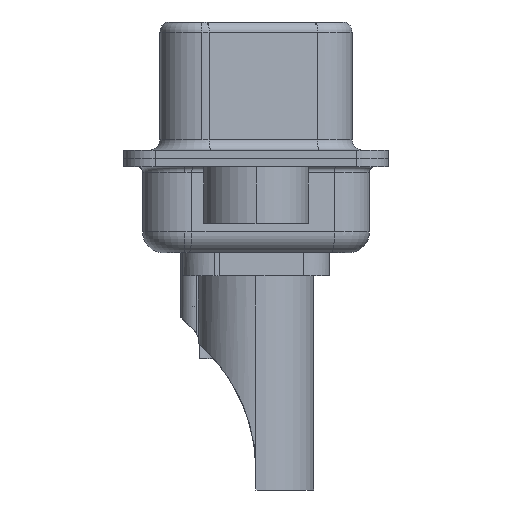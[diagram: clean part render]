
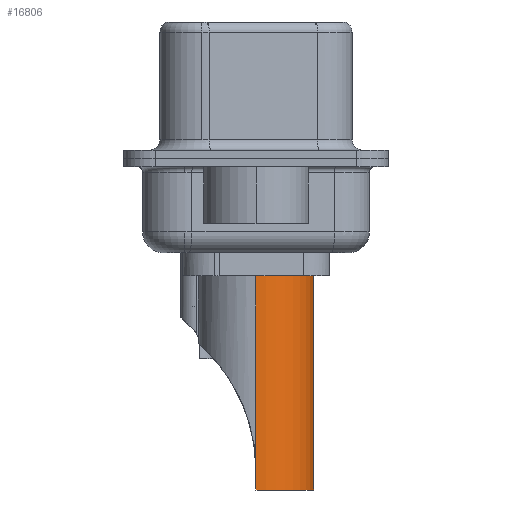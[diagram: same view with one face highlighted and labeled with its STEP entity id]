
A CAD part, left-side view. The second image highlights one B-rep face of the part: STEP entity #16806.
In plain terms, the highlighted cylindrical face has radius 2.75 mm (diameter 5.5 mm), a partial arc.
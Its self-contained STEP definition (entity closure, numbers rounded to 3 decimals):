
#46 = CARTESIAN_POINT ( 'NONE',  ( -2.75, 0., -8.7 ) ) ;
#313 = DIRECTION ( 'NONE',  ( 1., 0., 0. ) ) ;
#551 = VECTOR ( 'NONE', #22074, 1000. ) ;
#623 = VERTEX_POINT ( 'NONE', #10747 ) ;
#1064 = VERTEX_POINT ( 'NONE', #5358 ) ;
#1461 = EDGE_CURVE ( 'NONE', #8605, #7674, #19574, .T. ) ;
#1521 = VECTOR ( 'NONE', #18967, 1000. ) ;
#2049 = EDGE_CURVE ( 'NONE', #623, #7674, #20118, .T. ) ;
#2072 = DIRECTION ( 'NONE',  ( 0., 0., 1. ) ) ;
#3609 = CYLINDRICAL_SURFACE ( 'NONE', #22274, 2.75 ) ;
#4713 = ORIENTED_EDGE ( 'NONE', *, *, #18797, .T. ) ;
#4918 = LINE ( 'NONE', #21689, #9690 ) ;
#4948 = DIRECTION ( 'NONE',  ( 0., 0., 1. ) ) ;
#5270 = LINE ( 'NONE', #18436, #551 ) ;
#5358 = CARTESIAN_POINT ( 'NONE',  ( -2.75, 0., -7.764 ) ) ;
#5475 = DIRECTION ( 'NONE',  ( 0., 0., -1. ) ) ;
#7674 = VERTEX_POINT ( 'NONE', #19712 ) ;
#7892 = EDGE_CURVE ( 'NONE', #623, #22206, #5270, .T. ) ;
#8605 = VERTEX_POINT ( 'NONE', #18843 ) ;
#8950 = FACE_OUTER_BOUND ( 'NONE', #19114, .T. ) ;
#9690 = VECTOR ( 'NONE', #5475, 1000. ) ;
#9710 = ORIENTED_EDGE ( 'NONE', *, *, #7892, .F. ) ;
#9811 = CARTESIAN_POINT ( 'NONE',  ( -2.75, 0., 4.234 ) ) ;
#9864 = DIRECTION ( 'NONE',  ( 0., 0., 1. ) ) ;
#9958 = ORIENTED_EDGE ( 'NONE', *, *, #2049, .T. ) ;
#10747 = CARTESIAN_POINT ( 'NONE',  ( 2.75, 0., -7.764 ) ) ;
#11402 = CARTESIAN_POINT ( 'NONE',  ( 2.75, 0., 4.234 ) ) ;
#14453 = EDGE_CURVE ( 'NONE', #1064, #8605, #18076, .T. ) ;
#14494 = AXIS2_PLACEMENT_3D ( 'NONE', #16357, #4948, #313 ) ;
#14558 = DIRECTION ( 'NONE',  ( 1., 0., 0. ) ) ;
#15108 = EDGE_CURVE ( 'NONE', #21601, #22206, #22871, .T. ) ;
#16357 = CARTESIAN_POINT ( 'NONE',  ( 0., 0., 1.5 ) ) ;
#16462 = AXIS2_PLACEMENT_3D ( 'NONE', #20725, #9864, #22537 ) ;
#16806 = ADVANCED_FACE ( 'NONE', ( #8950 ), #3609, .T. ) ;
#18076 = LINE ( 'NONE', #9811, #22335 ) ;
#18240 = ORIENTED_EDGE ( 'NONE', *, *, #15108, .T. ) ;
#18436 = CARTESIAN_POINT ( 'NONE',  ( 2.75, 0., -8.7 ) ) ;
#18591 = ORIENTED_EDGE ( 'NONE', *, *, #1461, .F. ) ;
#18674 = CARTESIAN_POINT ( 'NONE',  ( 2.75, 0., -8.7 ) ) ;
#18797 = EDGE_CURVE ( 'NONE', #1064, #21601, #4918, .T. ) ;
#18843 = CARTESIAN_POINT ( 'NONE',  ( -2.75, 0., 1.5 ) ) ;
#18967 = DIRECTION ( 'NONE',  ( 0., 0., 1. ) ) ;
#19114 = EDGE_LOOP ( 'NONE', ( #20488, #4713, #18240, #9710, #9958, #18591 ) ) ;
#19574 = CIRCLE ( 'NONE', #14494, 2.75 ) ;
#19712 = CARTESIAN_POINT ( 'NONE',  ( 2.75, 0., 1.5 ) ) ;
#20118 = LINE ( 'NONE', #11402, #1521 ) ;
#20488 = ORIENTED_EDGE ( 'NONE', *, *, #14453, .F. ) ;
#20725 = CARTESIAN_POINT ( 'NONE',  ( 0., 0., -8.7 ) ) ;
#21601 = VERTEX_POINT ( 'NONE', #46 ) ;
#21689 = CARTESIAN_POINT ( 'NONE',  ( -2.75, 0., -8.7 ) ) ;
#21829 = CARTESIAN_POINT ( 'NONE',  ( 0., 0., 4.234 ) ) ;
#22074 = DIRECTION ( 'NONE',  ( 0., 0., -1. ) ) ;
#22206 = VERTEX_POINT ( 'NONE', #18674 ) ;
#22274 = AXIS2_PLACEMENT_3D ( 'NONE', #21829, #2072, #14558 ) ;
#22335 = VECTOR ( 'NONE', #22478, 1000. ) ;
#22478 = DIRECTION ( 'NONE',  ( 0., 0., 1. ) ) ;
#22537 = DIRECTION ( 'NONE',  ( 1., 0., 0. ) ) ;
#22871 = CIRCLE ( 'NONE', #16462, 2.75 ) ;
